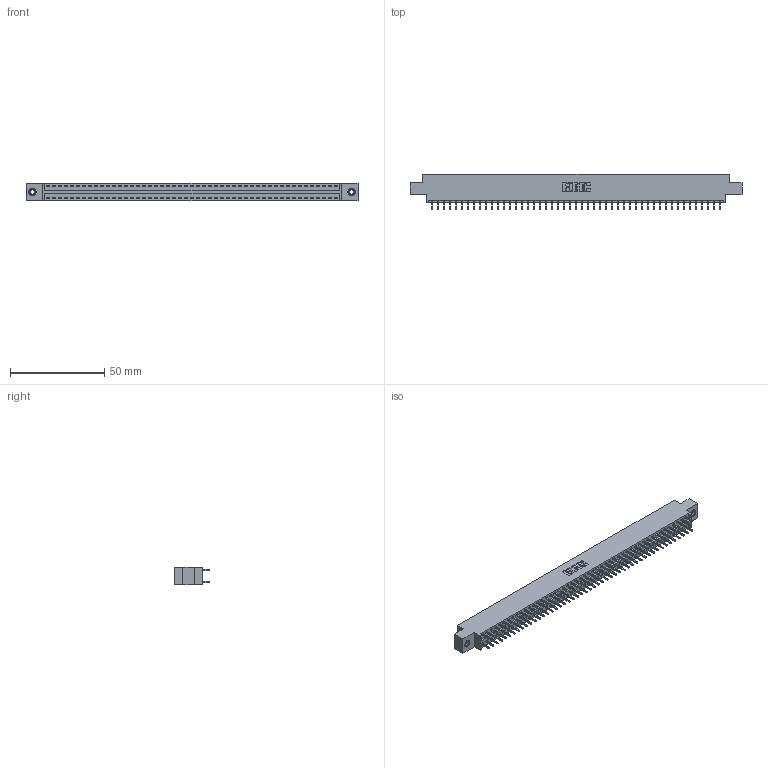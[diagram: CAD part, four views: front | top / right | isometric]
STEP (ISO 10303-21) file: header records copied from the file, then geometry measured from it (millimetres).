
FILE_DESCRIPTION (( 'STEP AP203' ), '1' );
FILE_NAME ('396-098-521-808.STEP', '2019-11-02T16:59:02', ( '' ), ( '' ), 'SwSTEP 2.0', 'SolidWorks 2016', '' );
FILE_SCHEMA (( 'CONFIG_CONTROL_DESIGN' ));
Length unit declared in the file: inch
Products named in the file (4): 346 Part_0.170 Offset - 0.156 Dia-TI; 345-292-001_345-293-121; 345-250-001_345-250-003-102; 396-098-521-808
Assembly tree (101 placements, depth 2):
  396-098-521-808
    346 Part_0.170 Offset - 0.156 Dia-TI
    345-292-001_345-293-121  x98
    345-250-001_345-250-003-102  x2
Bounding box: 176.15 x 19.05 x 9.4 mm (x, y, z)
Volume: 17030 mm3; surface area: 23449.1 mm2
Topology: 101 solids, 101 shells, 5282 faces, 15667 edges, 10306 vertices
Faces by surface type: plane 3542, cylinder 1724, cone 12, torus 4
Entity records: 32372 total; most frequent: CARTESIAN_POINT 5311, ORIENTED_EDGE 5238, DIRECTION 4757, EDGE_CURVE 2619, VECTOR 2271, LINE 2271, VERTEX_POINT 1740, AXIS2_PLACEMENT_3D 1243
